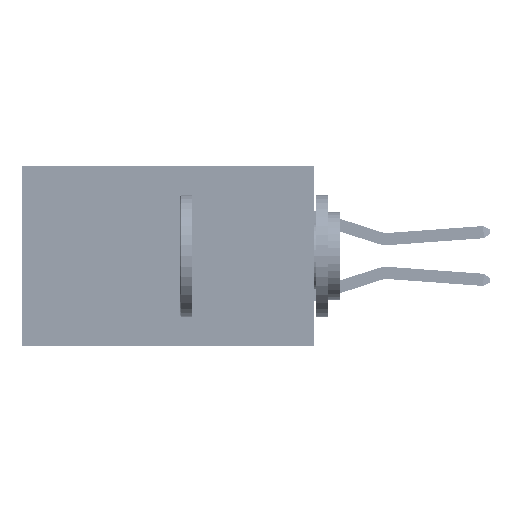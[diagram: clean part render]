
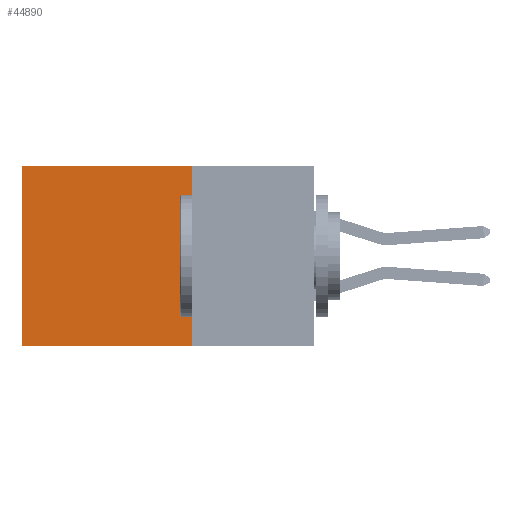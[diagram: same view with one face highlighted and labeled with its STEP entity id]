
A CAD part, left-side view. The second image highlights one B-rep face of the part: STEP entity #44890.
In plain terms, the highlighted planar face has unit normal (-1, 0, 0).
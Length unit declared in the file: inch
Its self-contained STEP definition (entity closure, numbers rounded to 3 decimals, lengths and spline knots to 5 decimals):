
#240 = EDGE_CURVE ( 'NONE', #35975, #26812, #13215, .T. ) ;
#4502 = LINE ( 'NONE', #18232, #12838 ) ;
#5380 = CARTESIAN_POINT ( 'NONE',  ( 0.2875, 0.25, -0.37 ) ) ;
#6746 = VECTOR ( 'NONE', #42016, 39.37008 ) ;
#6798 = CARTESIAN_POINT ( 'NONE',  ( 0.2875, 0.25, -0.37 ) ) ;
#7864 = LINE ( 'NONE', #31592, #6746 ) ;
#10391 = DIRECTION ( 'NONE',  ( 0., 1., 0. ) ) ;
#10646 = ORIENTED_EDGE ( 'NONE', *, *, #240, .F. ) ;
#11623 = FACE_OUTER_BOUND ( 'NONE', #33722, .T. ) ;
#12838 = VECTOR ( 'NONE', #29020, 39.37008 ) ;
#13215 = LINE ( 'NONE', #32749, #30849 ) ;
#13306 = EDGE_CURVE ( 'NONE', #16510, #30150, #7864, .T. ) ;
#13892 = PLANE ( 'NONE',  #19414 ) ;
#15212 = CARTESIAN_POINT ( 'NONE',  ( 0.2875, 0.6, 0. ) ) ;
#16510 = VERTEX_POINT ( 'NONE', #15212 ) ;
#17299 = CARTESIAN_POINT ( 'NONE',  ( 0.2875, 0.25, 0. ) ) ;
#17455 = DIRECTION ( 'NONE',  ( 1., 0., 0. ) ) ;
#18232 = CARTESIAN_POINT ( 'NONE',  ( 0.2875, 0.25, 0. ) ) ;
#19414 = AXIS2_PLACEMENT_3D ( 'NONE', #17299, #17455, #41836 ) ;
#20319 = CARTESIAN_POINT ( 'NONE',  ( 0.2875, 0.6, -0.37 ) ) ;
#21874 = ORIENTED_EDGE ( 'NONE', *, *, #40351, .T. ) ;
#22647 = ORIENTED_EDGE ( 'NONE', *, *, #13306, .T. ) ;
#25013 = ORIENTED_EDGE ( 'NONE', *, *, #32169, .F. ) ;
#26812 = VERTEX_POINT ( 'NONE', #5380 ) ;
#27657 = CARTESIAN_POINT ( 'NONE',  ( 0.2875, 0.25, 0. ) ) ;
#29020 = DIRECTION ( 'NONE',  ( 0., 1., 0. ) ) ;
#30150 = VERTEX_POINT ( 'NONE', #20319 ) ;
#30849 = VECTOR ( 'NONE', #36243, 39.37008 ) ;
#31592 = CARTESIAN_POINT ( 'NONE',  ( 0.2875, 0.6, 0. ) ) ;
#32169 = EDGE_CURVE ( 'NONE', #26812, #30150, #39372, .T. ) ;
#32749 = CARTESIAN_POINT ( 'NONE',  ( 0.2875, 0.25, 0. ) ) ;
#33722 = EDGE_LOOP ( 'NONE', ( #22647, #25013, #10646, #21874 ) ) ;
#35975 = VERTEX_POINT ( 'NONE', #27657 ) ;
#36243 = DIRECTION ( 'NONE',  ( 0., 0., -1. ) ) ;
#38300 = VECTOR ( 'NONE', #10391, 39.37008 ) ;
#39372 = LINE ( 'NONE', #6798, #38300 ) ;
#40351 = EDGE_CURVE ( 'NONE', #35975, #16510, #4502, .T. ) ;
#41836 = DIRECTION ( 'NONE',  ( 0., 0., -1. ) ) ;
#42016 = DIRECTION ( 'NONE',  ( 0., 0., -1. ) ) ;
#44890 = ADVANCED_FACE ( 'NONE', ( #11623 ), #13892, .F. ) ;
